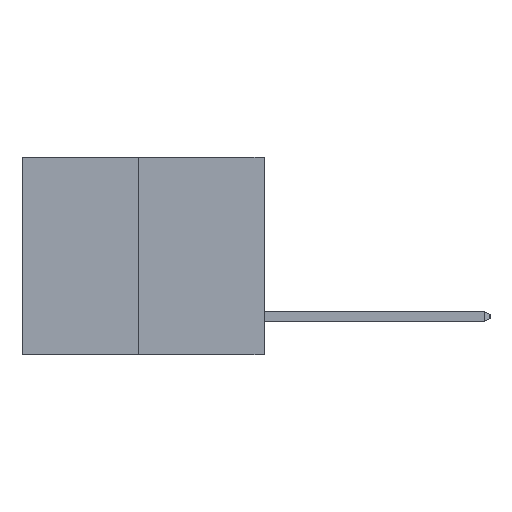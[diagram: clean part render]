
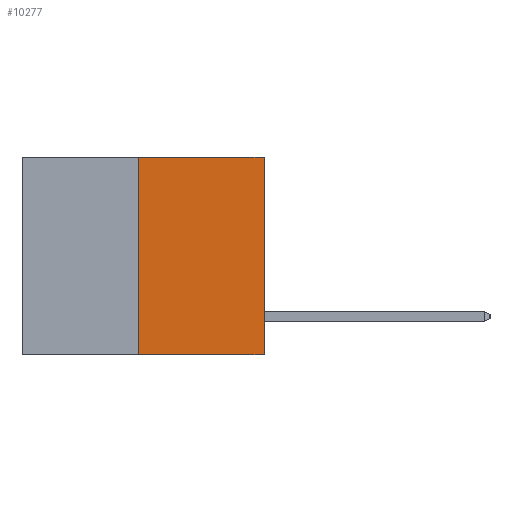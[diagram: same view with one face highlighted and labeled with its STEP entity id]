
A CAD part, left-side view. The second image highlights one B-rep face of the part: STEP entity #10277.
In plain terms, the highlighted planar face has unit normal (-1, 0, 0).
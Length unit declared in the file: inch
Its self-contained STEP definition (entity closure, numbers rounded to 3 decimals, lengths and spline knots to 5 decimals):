
#69 = VECTOR ( 'NONE', #7332, 39.37008 ) ;
#330 = CARTESIAN_POINT ( 'NONE',  ( 0., 0.6, 0. ) ) ;
#778 = CARTESIAN_POINT ( 'NONE',  ( 0., 0.312, -0.49 ) ) ;
#788 = LINE ( 'NONE', #9748, #2123 ) ;
#829 = CARTESIAN_POINT ( 'NONE',  ( 0., 0., -0.49 ) ) ;
#1432 = DIRECTION ( 'NONE',  ( 0., 0., 1. ) ) ;
#1513 = CARTESIAN_POINT ( 'NONE',  ( 0., 0., 0. ) ) ;
#1619 = LINE ( 'NONE', #7214, #3836 ) ;
#1859 = VERTEX_POINT ( 'NONE', #829 ) ;
#2074 = DIRECTION ( 'NONE',  ( 0., -1., 0. ) ) ;
#2123 = VECTOR ( 'NONE', #2074, 39.37008 ) ;
#2397 = DIRECTION ( 'NONE',  ( 0., 0., 1. ) ) ;
#2597 = LINE ( 'NONE', #330, #69 ) ;
#2932 = VECTOR ( 'NONE', #1432, 39.37008 ) ;
#3363 = ORIENTED_EDGE ( 'NONE', *, *, #4346, .F. ) ;
#3836 = VECTOR ( 'NONE', #2397, 39.37008 ) ;
#4145 = LINE ( 'NONE', #1513, #2932 ) ;
#4344 = VERTEX_POINT ( 'NONE', #7467 ) ;
#4346 = EDGE_CURVE ( 'NONE', #9178, #4344, #1619, .T. ) ;
#5566 = EDGE_CURVE ( 'NONE', #4344, #11806, #2597, .T. ) ;
#6242 = ORIENTED_EDGE ( 'NONE', *, *, #6267, .T. ) ;
#6267 = EDGE_CURVE ( 'NONE', #9178, #1859, #788, .T. ) ;
#6402 = PLANE ( 'NONE',  #9348 ) ;
#6558 = EDGE_LOOP ( 'NONE', ( #3363, #6242, #9986, #10903 ) ) ;
#7214 = CARTESIAN_POINT ( 'NONE',  ( 0., 0.312, -0.49 ) ) ;
#7281 = DIRECTION ( 'NONE',  ( 0., 0., -1. ) ) ;
#7332 = DIRECTION ( 'NONE',  ( 0., -1., 0. ) ) ;
#7467 = CARTESIAN_POINT ( 'NONE',  ( 0., 0.312, 0. ) ) ;
#8262 = CARTESIAN_POINT ( 'NONE',  ( 0., 0.6, 0. ) ) ;
#9028 = CARTESIAN_POINT ( 'NONE',  ( 0., 0., 0. ) ) ;
#9178 = VERTEX_POINT ( 'NONE', #778 ) ;
#9348 = AXIS2_PLACEMENT_3D ( 'NONE', #8262, #11255, #7281 ) ;
#9637 = FACE_OUTER_BOUND ( 'NONE', #6558, .T. ) ;
#9748 = CARTESIAN_POINT ( 'NONE',  ( 0., 0.6, -0.49 ) ) ;
#9986 = ORIENTED_EDGE ( 'NONE', *, *, #11369, .T. ) ;
#10277 = ADVANCED_FACE ( 'NONE', ( #9637 ), #6402, .F. ) ;
#10903 = ORIENTED_EDGE ( 'NONE', *, *, #5566, .F. ) ;
#11255 = DIRECTION ( 'NONE',  ( 1., 0., 0. ) ) ;
#11369 = EDGE_CURVE ( 'NONE', #1859, #11806, #4145, .T. ) ;
#11806 = VERTEX_POINT ( 'NONE', #9028 ) ;
